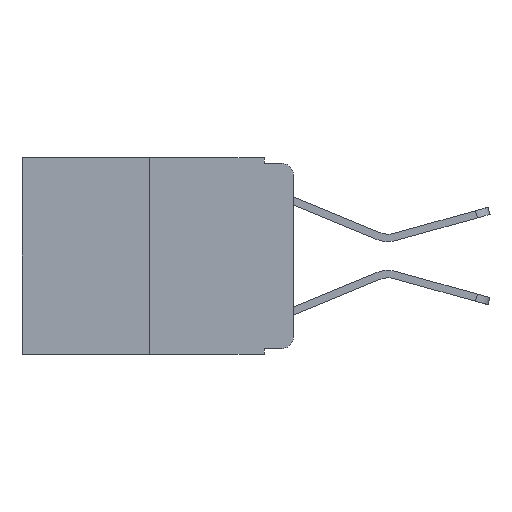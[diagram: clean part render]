
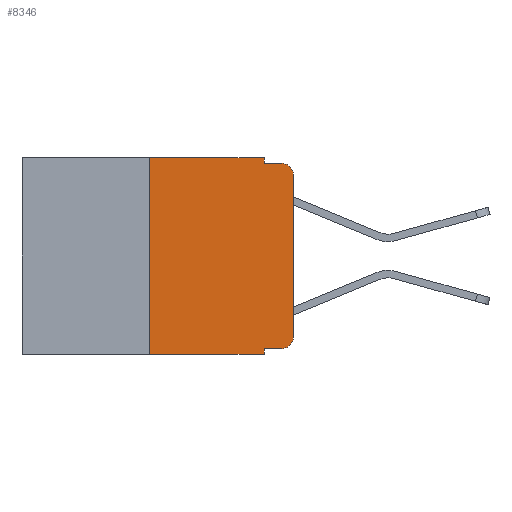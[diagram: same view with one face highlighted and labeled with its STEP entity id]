
A CAD part, left-side view. The second image highlights one B-rep face of the part: STEP entity #8346.
In plain terms, the highlighted planar face has unit normal (-1, 0, 0).
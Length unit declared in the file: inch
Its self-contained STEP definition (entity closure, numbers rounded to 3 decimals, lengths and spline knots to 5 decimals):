
#34 = EDGE_CURVE ( 'NONE', #12174, #13911, #3987, .T. ) ;
#59 = DIRECTION ( 'NONE',  ( -1., 0., 0. ) ) ;
#85 = LINE ( 'NONE', #2276, #3462 ) ;
#243 = VECTOR ( 'NONE', #9340, 39.37008 ) ;
#517 = ORIENTED_EDGE ( 'NONE', *, *, #11065, .F. ) ;
#629 = CARTESIAN_POINT ( 'NONE',  ( 0., 0.051, -0.01 ) ) ;
#796 = PLANE ( 'NONE',  #14628 ) ;
#987 = DIRECTION ( 'NONE',  ( 0., -1., 0. ) ) ;
#1607 = CARTESIAN_POINT ( 'NONE',  ( 0., 0.051, -0.333 ) ) ;
#2039 = DIRECTION ( 'NONE',  ( 0., 0., 1. ) ) ;
#2062 = EDGE_CURVE ( 'NONE', #7666, #5138, #9530, .T. ) ;
#2276 = CARTESIAN_POINT ( 'NONE',  ( 0., 0.051, 0. ) ) ;
#2324 = VECTOR ( 'NONE', #987, 39.37008 ) ;
#2469 = CARTESIAN_POINT ( 'NONE',  ( 0., 0.473, 0. ) ) ;
#2808 = CARTESIAN_POINT ( 'NONE',  ( 0., 0.473, -0.343 ) ) ;
#2860 = EDGE_CURVE ( 'NONE', #15722, #14582, #8927, .T. ) ;
#2985 = EDGE_CURVE ( 'NONE', #5970, #5138, #10262, .T. ) ;
#3094 = VERTEX_POINT ( 'NONE', #6476 ) ;
#3350 = LINE ( 'NONE', #14415, #9921 ) ;
#3462 = VECTOR ( 'NONE', #8476, 39.37008 ) ;
#3620 = LINE ( 'NONE', #10565, #243 ) ;
#3987 = LINE ( 'NONE', #9156, #13437 ) ;
#4067 = VERTEX_POINT ( 'NONE', #15657 ) ;
#4076 = VERTEX_POINT ( 'NONE', #14505 ) ;
#4302 = FACE_OUTER_BOUND ( 'NONE', #15452, .T. ) ;
#5138 = VERTEX_POINT ( 'NONE', #15572 ) ;
#5928 = CARTESIAN_POINT ( 'NONE',  ( 0., 0.25, -0.343 ) ) ;
#5970 = VERTEX_POINT ( 'NONE', #9326 ) ;
#6476 = CARTESIAN_POINT ( 'NONE',  ( 0., 0.051, -0.343 ) ) ;
#6973 = DIRECTION ( 'NONE',  ( -1., 0., 0. ) ) ;
#7117 = DIRECTION ( 'NONE',  ( 0., 0., -1. ) ) ;
#7497 = EDGE_CURVE ( 'NONE', #4076, #5970, #3350, .T. ) ;
#7566 = CARTESIAN_POINT ( 'NONE',  ( 0., 0.02, -0.03 ) ) ;
#7666 = VERTEX_POINT ( 'NONE', #8615 ) ;
#7853 = EDGE_CURVE ( 'NONE', #12174, #3094, #14708, .T. ) ;
#8156 = ORIENTED_EDGE ( 'NONE', *, *, #2985, .T. ) ;
#8179 = VECTOR ( 'NONE', #13592, 39.37008 ) ;
#8346 = ADVANCED_FACE ( 'NONE', ( #4302 ), #796, .F. ) ;
#8454 = CARTESIAN_POINT ( 'NONE',  ( 0., 0.02, -0.333 ) ) ;
#8473 = CARTESIAN_POINT ( 'NONE',  ( 0., 0.051, -0.333 ) ) ;
#8476 = DIRECTION ( 'NONE',  ( 0., 0., -1. ) ) ;
#8517 = EDGE_CURVE ( 'NONE', #13911, #4067, #14711, .T. ) ;
#8538 = ORIENTED_EDGE ( 'NONE', *, *, #2062, .F. ) ;
#8615 = CARTESIAN_POINT ( 'NONE',  ( 0., 0.051, -0.01 ) ) ;
#8787 = DIRECTION ( 'NONE',  ( 0., 0., -1. ) ) ;
#8927 = LINE ( 'NONE', #8473, #2324 ) ;
#8983 = DIRECTION ( 'NONE',  ( 0., -1., 0. ) ) ;
#9156 = CARTESIAN_POINT ( 'NONE',  ( 0., 0.25, 0. ) ) ;
#9304 = ORIENTED_EDGE ( 'NONE', *, *, #8517, .F. ) ;
#9326 = CARTESIAN_POINT ( 'NONE',  ( 0., 0., -0.03 ) ) ;
#9340 = DIRECTION ( 'NONE',  ( 0., 0., -1. ) ) ;
#9364 = DIRECTION ( 'NONE',  ( 0., -1., 0. ) ) ;
#9530 = LINE ( 'NONE', #629, #12794 ) ;
#9921 = VECTOR ( 'NONE', #2039, 39.37008 ) ;
#10081 = ORIENTED_EDGE ( 'NONE', *, *, #7853, .T. ) ;
#10262 = CIRCLE ( 'NONE', #12503, 0.02 ) ;
#10452 = ORIENTED_EDGE ( 'NONE', *, *, #2860, .T. ) ;
#10565 = CARTESIAN_POINT ( 'NONE',  ( 0., 0.051, 0. ) ) ;
#10857 = ORIENTED_EDGE ( 'NONE', *, *, #13909, .T. ) ;
#11065 = EDGE_CURVE ( 'NONE', #15722, #3094, #85, .T. ) ;
#11859 = CARTESIAN_POINT ( 'NONE',  ( 0., 0.25, 0. ) ) ;
#12004 = CARTESIAN_POINT ( 'NONE',  ( 0., 0.473, 0. ) ) ;
#12117 = AXIS2_PLACEMENT_3D ( 'NONE', #14301, #6973, #15523 ) ;
#12174 = VERTEX_POINT ( 'NONE', #5928 ) ;
#12465 = CIRCLE ( 'NONE', #12117, 0.02 ) ;
#12503 = AXIS2_PLACEMENT_3D ( 'NONE', #7566, #59, #8787 ) ;
#12574 = ORIENTED_EDGE ( 'NONE', *, *, #34, .F. ) ;
#12794 = VECTOR ( 'NONE', #9364, 39.37008 ) ;
#13246 = EDGE_CURVE ( 'NONE', #4067, #7666, #3620, .T. ) ;
#13437 = VECTOR ( 'NONE', #15260, 39.37008 ) ;
#13592 = DIRECTION ( 'NONE',  ( 0., -1., 0. ) ) ;
#13909 = EDGE_CURVE ( 'NONE', #14582, #4076, #12465, .T. ) ;
#13911 = VERTEX_POINT ( 'NONE', #11859 ) ;
#13920 = VECTOR ( 'NONE', #8983, 39.37008 ) ;
#14283 = ORIENTED_EDGE ( 'NONE', *, *, #7497, .T. ) ;
#14301 = CARTESIAN_POINT ( 'NONE',  ( 0., 0.02, -0.313 ) ) ;
#14415 = CARTESIAN_POINT ( 'NONE',  ( 0., 0., 0. ) ) ;
#14456 = DIRECTION ( 'NONE',  ( 1., 0., 0. ) ) ;
#14505 = CARTESIAN_POINT ( 'NONE',  ( 0., 0., -0.313 ) ) ;
#14582 = VERTEX_POINT ( 'NONE', #8454 ) ;
#14628 = AXIS2_PLACEMENT_3D ( 'NONE', #12004, #14456, #7117 ) ;
#14708 = LINE ( 'NONE', #2808, #13920 ) ;
#14711 = LINE ( 'NONE', #2469, #8179 ) ;
#15048 = ORIENTED_EDGE ( 'NONE', *, *, #13246, .F. ) ;
#15260 = DIRECTION ( 'NONE',  ( 0., 0., 1. ) ) ;
#15452 = EDGE_LOOP ( 'NONE', ( #14283, #8156, #8538, #15048, #9304, #12574, #10081, #517, #10452, #10857 ) ) ;
#15523 = DIRECTION ( 'NONE',  ( 0., 0., -1. ) ) ;
#15572 = CARTESIAN_POINT ( 'NONE',  ( 0., 0.02, -0.01 ) ) ;
#15657 = CARTESIAN_POINT ( 'NONE',  ( 0., 0.051, 0. ) ) ;
#15722 = VERTEX_POINT ( 'NONE', #1607 ) ;
